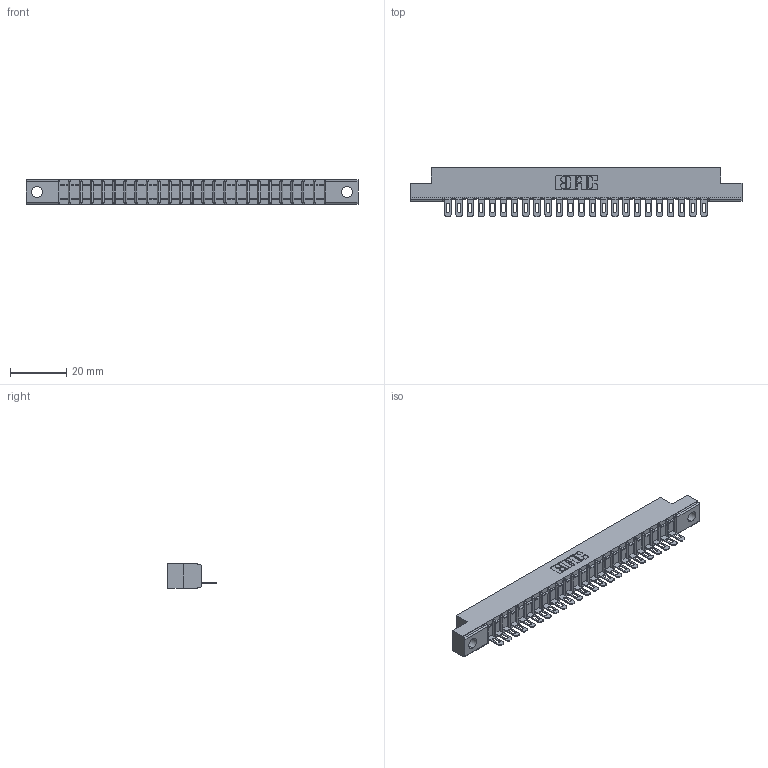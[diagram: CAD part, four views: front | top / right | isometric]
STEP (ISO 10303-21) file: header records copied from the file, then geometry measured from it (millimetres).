
FILE_DESCRIPTION (( 'STEP AP203' ), '1' );
FILE_NAME ('307-024-501-102.STEP', '2018-08-04T06:19:12', ( '' ), ( '' ), 'SwSTEP 2.0', 'SolidWorks 2016', '' );
FILE_SCHEMA (( 'CONFIG_CONTROL_DESIGN' ));
Length unit declared in the file: inch
Products named in the file (3): 307 Part_.128 Dia Mounting Holes; 307-290-002_501; 307-024-501-102
Assembly tree (25 placements, depth 2):
  307-024-501-102
    307 Part_.128 Dia Mounting Holes
    307-290-002_501  x24
Bounding box: 118.11 x 17.42 x 8.71 mm (x, y, z)
Volume: 7731.5 mm3; surface area: 14183.2 mm2
Topology: 25 solids, 25 shells, 1967 faces, 6035 edges, 3954 vertices
Faces by surface type: plane 1126, cylinder 791, sphere 50
Entity records: 23590 total; most frequent: CARTESIAN_POINT 3976, ORIENTED_EDGE 3966, DIRECTION 3875, EDGE_CURVE 1983, LINE 1505, VECTOR 1505, VERTEX_POINT 1286, AXIS2_PLACEMENT_3D 1185
